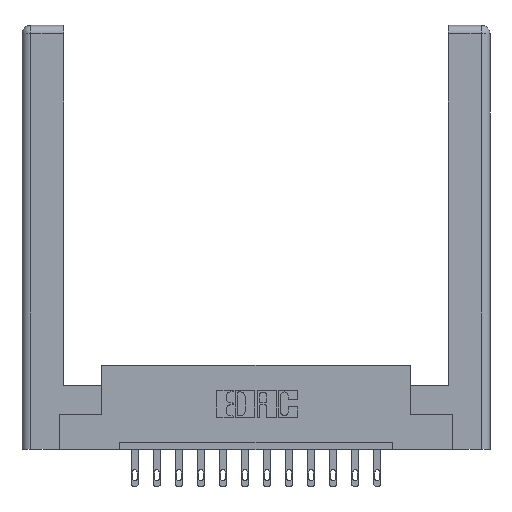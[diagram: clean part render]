
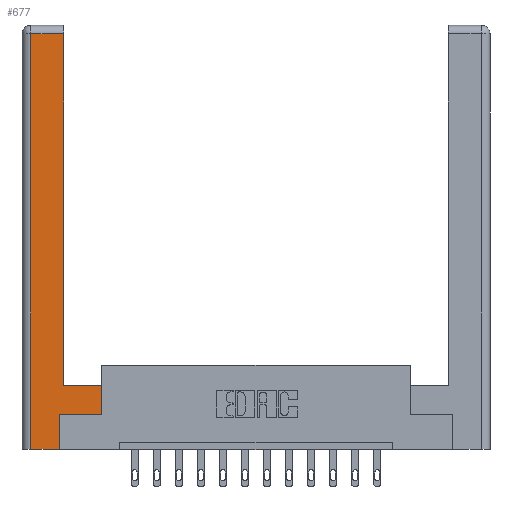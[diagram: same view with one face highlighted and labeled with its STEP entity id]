
A CAD part, top view. The second image highlights one B-rep face of the part: STEP entity #677.
In plain terms, the highlighted planar face has unit normal (0, 0, 1).
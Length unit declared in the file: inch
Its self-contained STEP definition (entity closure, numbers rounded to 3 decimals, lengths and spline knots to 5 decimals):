
#115 = DIRECTION ( 'NONE',  ( 0., 0., -1. ) ) ;
#237 = CARTESIAN_POINT ( 'NONE',  ( 0.565, 0.245, 0. ) ) ;
#380 = CARTESIAN_POINT ( 'NONE',  ( 0.265, 0., 0. ) ) ;
#638 = FACE_OUTER_BOUND ( 'NONE', #12756, .T. ) ;
#677 = ADVANCED_FACE ( 'NONE', ( #638 ), #5969, .F. ) ;
#755 = VECTOR ( 'NONE', #7330, 39.37008 ) ;
#1223 = EDGE_CURVE ( 'NONE', #3344, #1612, #13818, .T. ) ;
#1390 = VERTEX_POINT ( 'NONE', #11337 ) ;
#1612 = VERTEX_POINT ( 'NONE', #5893 ) ;
#1729 = ORIENTED_EDGE ( 'NONE', *, *, #1223, .T. ) ;
#1931 = CARTESIAN_POINT ( 'NONE',  ( 0.565, 0.245, 0. ) ) ;
#2255 = VECTOR ( 'NONE', #8298, 39.37008 ) ;
#2417 = CARTESIAN_POINT ( 'NONE',  ( 0.295, 3., 0. ) ) ;
#3019 = DIRECTION ( 'NONE',  ( 0., -1., 0. ) ) ;
#3134 = CARTESIAN_POINT ( 'NONE',  ( 0.295, 0.45, 0. ) ) ;
#3344 = VERTEX_POINT ( 'NONE', #1931 ) ;
#3361 = EDGE_CURVE ( 'NONE', #11276, #8002, #7565, .T. ) ;
#3769 = DIRECTION ( 'NONE',  ( 1., 0., 0. ) ) ;
#3944 = ORIENTED_EDGE ( 'NONE', *, *, #4877, .T. ) ;
#4324 = CARTESIAN_POINT ( 'NONE',  ( 0.0615, 0., 0. ) ) ;
#4433 = ORIENTED_EDGE ( 'NONE', *, *, #14456, .T. ) ;
#4657 = VECTOR ( 'NONE', #10958, 39.37008 ) ;
#4788 = CARTESIAN_POINT ( 'NONE',  ( 0.295, 0.45, 0. ) ) ;
#4877 = EDGE_CURVE ( 'NONE', #1390, #7274, #7178, .T. ) ;
#4983 = DIRECTION ( 'NONE',  ( 0., 1., 0. ) ) ;
#5410 = CARTESIAN_POINT ( 'NONE',  ( 0.0615, 0., 0. ) ) ;
#5729 = ORIENTED_EDGE ( 'NONE', *, *, #3361, .T. ) ;
#5834 = CARTESIAN_POINT ( 'NONE',  ( 0.265, 0.245, 0. ) ) ;
#5893 = CARTESIAN_POINT ( 'NONE',  ( 0.565, 0.45, 0. ) ) ;
#5969 = PLANE ( 'NONE',  #6579 ) ;
#5989 = ORIENTED_EDGE ( 'NONE', *, *, #13406, .T. ) ;
#6021 = DIRECTION ( 'NONE',  ( -1., 0., 0. ) ) ;
#6048 = ORIENTED_EDGE ( 'NONE', *, *, #13911, .T. ) ;
#6445 = VECTOR ( 'NONE', #3019, 39.37008 ) ;
#6579 = AXIS2_PLACEMENT_3D ( 'NONE', #14281, #115, #6021 ) ;
#6720 = LINE ( 'NONE', #2417, #2255 ) ;
#7178 = LINE ( 'NONE', #5834, #9248 ) ;
#7192 = EDGE_CURVE ( 'NONE', #10754, #10601, #6720, .T. ) ;
#7274 = VERTEX_POINT ( 'NONE', #14117 ) ;
#7330 = DIRECTION ( 'NONE',  ( -1., 0., 0. ) ) ;
#7565 = LINE ( 'NONE', #4324, #6445 ) ;
#7820 = EDGE_CURVE ( 'NONE', #10601, #11276, #14691, .T. ) ;
#8002 = VERTEX_POINT ( 'NONE', #5410 ) ;
#8298 = DIRECTION ( 'NONE',  ( 0., 1., 0. ) ) ;
#9248 = VECTOR ( 'NONE', #10745, 39.37008 ) ;
#10031 = ORIENTED_EDGE ( 'NONE', *, *, #7820, .T. ) ;
#10601 = VERTEX_POINT ( 'NONE', #12711 ) ;
#10745 = DIRECTION ( 'NONE',  ( 0., 1., 0. ) ) ;
#10754 = VERTEX_POINT ( 'NONE', #3134 ) ;
#10787 = LINE ( 'NONE', #4788, #13366 ) ;
#10958 = DIRECTION ( 'NONE',  ( 1., 0., 0. ) ) ;
#11276 = VERTEX_POINT ( 'NONE', #11512 ) ;
#11337 = CARTESIAN_POINT ( 'NONE',  ( 0.265, 0., 0. ) ) ;
#11391 = LINE ( 'NONE', #237, #13225 ) ;
#11512 = CARTESIAN_POINT ( 'NONE',  ( 0.0615, 2.94, 0. ) ) ;
#11958 = VECTOR ( 'NONE', #4983, 39.37008 ) ;
#12079 = DIRECTION ( 'NONE',  ( -1., 0., 0. ) ) ;
#12550 = CARTESIAN_POINT ( 'NONE',  ( 0.565, 0.45, 0. ) ) ;
#12711 = CARTESIAN_POINT ( 'NONE',  ( 0.295, 2.94, 0. ) ) ;
#12756 = EDGE_LOOP ( 'NONE', ( #13737, #10031, #5729, #6048, #3944, #5989, #1729, #4433 ) ) ;
#13225 = VECTOR ( 'NONE', #3769, 39.37008 ) ;
#13256 = CARTESIAN_POINT ( 'NONE',  ( 0.0615, 2.94, 0. ) ) ;
#13366 = VECTOR ( 'NONE', #12079, 39.37008 ) ;
#13406 = EDGE_CURVE ( 'NONE', #7274, #3344, #11391, .T. ) ;
#13737 = ORIENTED_EDGE ( 'NONE', *, *, #7192, .T. ) ;
#13818 = LINE ( 'NONE', #12550, #11958 ) ;
#13911 = EDGE_CURVE ( 'NONE', #8002, #1390, #14502, .T. ) ;
#14117 = CARTESIAN_POINT ( 'NONE',  ( 0.265, 0.245, 0. ) ) ;
#14281 = CARTESIAN_POINT ( 'NONE',  ( 0., 0., 0. ) ) ;
#14456 = EDGE_CURVE ( 'NONE', #1612, #10754, #10787, .T. ) ;
#14502 = LINE ( 'NONE', #380, #4657 ) ;
#14691 = LINE ( 'NONE', #13256, #755 ) ;
